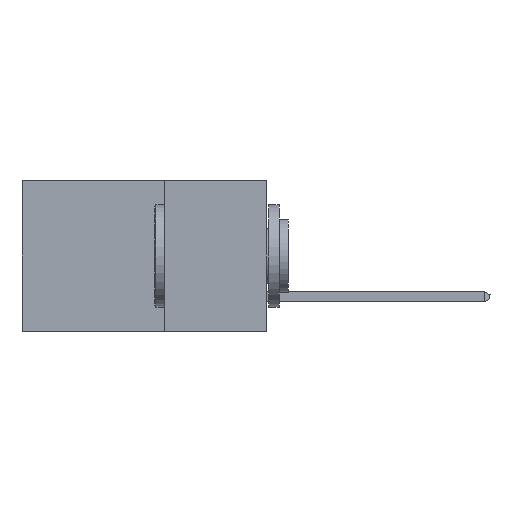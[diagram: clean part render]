
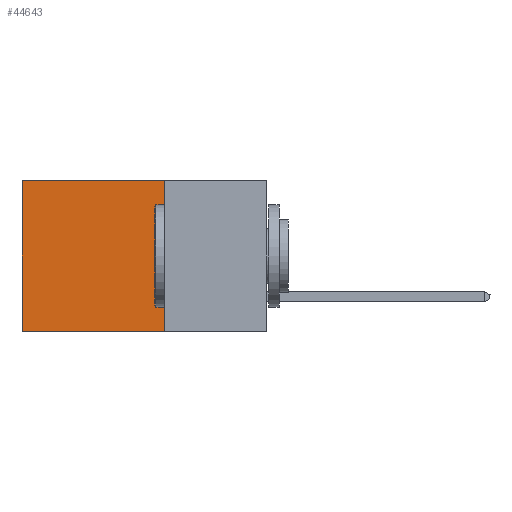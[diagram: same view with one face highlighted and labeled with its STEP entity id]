
A CAD part, left-side view. The second image highlights one B-rep face of the part: STEP entity #44643.
In plain terms, the highlighted planar face has unit normal (-1, 0, 0).
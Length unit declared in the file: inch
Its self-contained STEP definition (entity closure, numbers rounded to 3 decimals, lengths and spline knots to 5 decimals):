
#1336 = LINE ( 'NONE', #35236, #18789 ) ;
#3613 = EDGE_CURVE ( 'NONE', #27752, #11872, #3879, .T. ) ;
#3879 = LINE ( 'NONE', #18294, #15890 ) ;
#5249 = ORIENTED_EDGE ( 'NONE', *, *, #5585, .F. ) ;
#5585 = EDGE_CURVE ( 'NONE', #41745, #26781, #22278, .T. ) ;
#9770 = DIRECTION ( 'NONE',  ( 1., 0., 0. ) ) ;
#9951 = CARTESIAN_POINT ( 'NONE',  ( 0.2875, 0.6, -0.37 ) ) ;
#11872 = VERTEX_POINT ( 'NONE', #9951 ) ;
#13305 = DIRECTION ( 'NONE',  ( 0., 0., -1. ) ) ;
#14937 = EDGE_LOOP ( 'NONE', ( #26226, #36319, #5249, #24076 ) ) ;
#15890 = VECTOR ( 'NONE', #25389, 39.37008 ) ;
#15928 = CARTESIAN_POINT ( 'NONE',  ( 0.2875, 0.25, 0. ) ) ;
#17315 = VECTOR ( 'NONE', #18258, 39.37008 ) ;
#17577 = CARTESIAN_POINT ( 'NONE',  ( 0.2875, 0.25, 0. ) ) ;
#18258 = DIRECTION ( 'NONE',  ( 0., 1., 0. ) ) ;
#18294 = CARTESIAN_POINT ( 'NONE',  ( 0.2875, 0.6, 0. ) ) ;
#18789 = VECTOR ( 'NONE', #39202, 39.37008 ) ;
#20065 = VECTOR ( 'NONE', #37940, 39.37008 ) ;
#20113 = EDGE_CURVE ( 'NONE', #41745, #27752, #43548, .T. ) ;
#20189 = PLANE ( 'NONE',  #23357 ) ;
#22278 = LINE ( 'NONE', #17577, #20065 ) ;
#23357 = AXIS2_PLACEMENT_3D ( 'NONE', #44020, #9770, #13305 ) ;
#23594 = CARTESIAN_POINT ( 'NONE',  ( 0.2875, 0.6, 0. ) ) ;
#24076 = ORIENTED_EDGE ( 'NONE', *, *, #20113, .T. ) ;
#25389 = DIRECTION ( 'NONE',  ( 0., 0., -1. ) ) ;
#26226 = ORIENTED_EDGE ( 'NONE', *, *, #3613, .T. ) ;
#26781 = VERTEX_POINT ( 'NONE', #31883 ) ;
#27752 = VERTEX_POINT ( 'NONE', #23594 ) ;
#31883 = CARTESIAN_POINT ( 'NONE',  ( 0.2875, 0.25, -0.37 ) ) ;
#32728 = EDGE_CURVE ( 'NONE', #26781, #11872, #1336, .T. ) ;
#35236 = CARTESIAN_POINT ( 'NONE',  ( 0.2875, 0.25, -0.37 ) ) ;
#35715 = FACE_OUTER_BOUND ( 'NONE', #14937, .T. ) ;
#35877 = CARTESIAN_POINT ( 'NONE',  ( 0.2875, 0.25, 0. ) ) ;
#36319 = ORIENTED_EDGE ( 'NONE', *, *, #32728, .F. ) ;
#37940 = DIRECTION ( 'NONE',  ( 0., 0., -1. ) ) ;
#39202 = DIRECTION ( 'NONE',  ( 0., 1., 0. ) ) ;
#41745 = VERTEX_POINT ( 'NONE', #15928 ) ;
#43548 = LINE ( 'NONE', #35877, #17315 ) ;
#44020 = CARTESIAN_POINT ( 'NONE',  ( 0.2875, 0.25, 0. ) ) ;
#44643 = ADVANCED_FACE ( 'NONE', ( #35715 ), #20189, .F. ) ;
